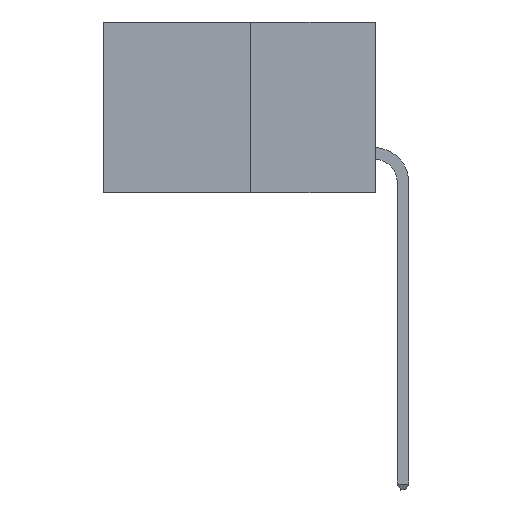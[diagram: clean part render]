
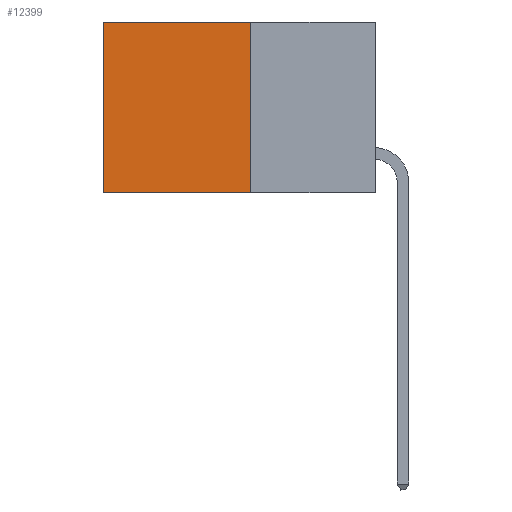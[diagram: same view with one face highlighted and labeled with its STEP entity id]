
A CAD part, left-side view. The second image highlights one B-rep face of the part: STEP entity #12399.
In plain terms, the highlighted planar face has unit normal (-1, 0, 0).
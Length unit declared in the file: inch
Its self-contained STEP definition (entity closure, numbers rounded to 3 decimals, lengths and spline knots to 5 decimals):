
#51 = LINE ( 'NONE', #8612, #17587 ) ;
#745 = FACE_OUTER_BOUND ( 'NONE', #1623, .T. ) ;
#1623 = EDGE_LOOP ( 'NONE', ( #15211, #9121, #4709, #14513 ) ) ;
#2615 = VERTEX_POINT ( 'NONE', #5876 ) ;
#2718 = VERTEX_POINT ( 'NONE', #7569 ) ;
#3143 = DIRECTION ( 'NONE',  ( 1., 0., 0. ) ) ;
#3274 = DIRECTION ( 'NONE',  ( 0., 1., 0. ) ) ;
#4709 = ORIENTED_EDGE ( 'NONE', *, *, #14621, .F. ) ;
#5876 = CARTESIAN_POINT ( 'NONE',  ( 0.277, 0.59, -0.37 ) ) ;
#6503 = CARTESIAN_POINT ( 'NONE',  ( 0.277, 0.59, -0.37 ) ) ;
#6609 = VECTOR ( 'NONE', #10995, 39.37008 ) ;
#7569 = CARTESIAN_POINT ( 'NONE',  ( 0.277, 0.27, -0.37 ) ) ;
#8198 = DIRECTION ( 'NONE',  ( 0., 0., -1. ) ) ;
#8321 = LINE ( 'NONE', #15035, #16805 ) ;
#8612 = CARTESIAN_POINT ( 'NONE',  ( 0.277, 0.27, 0. ) ) ;
#9121 = ORIENTED_EDGE ( 'NONE', *, *, #20484, .F. ) ;
#9159 = VERTEX_POINT ( 'NONE', #21028 ) ;
#10995 = DIRECTION ( 'NONE',  ( 0., 0., -1. ) ) ;
#11994 = DIRECTION ( 'NONE',  ( 0., 1., 0. ) ) ;
#12399 = ADVANCED_FACE ( 'NONE', ( #745 ), #20029, .F. ) ;
#13259 = CARTESIAN_POINT ( 'NONE',  ( 0.277, 0.27, -0.37 ) ) ;
#13660 = VECTOR ( 'NONE', #8198, 39.37008 ) ;
#14513 = ORIENTED_EDGE ( 'NONE', *, *, #18664, .T. ) ;
#14621 = EDGE_CURVE ( 'NONE', #21395, #2718, #20104, .T. ) ;
#14982 = DIRECTION ( 'NONE',  ( 0., 0., -1. ) ) ;
#15035 = CARTESIAN_POINT ( 'NONE',  ( 0.277, 0.27, -0.37 ) ) ;
#15211 = ORIENTED_EDGE ( 'NONE', *, *, #16924, .T. ) ;
#16805 = VECTOR ( 'NONE', #3274, 39.37008 ) ;
#16924 = EDGE_CURVE ( 'NONE', #9159, #2615, #18717, .T. ) ;
#17587 = VECTOR ( 'NONE', #11994, 39.37008 ) ;
#17857 = CARTESIAN_POINT ( 'NONE',  ( 0.277, 0.27, -0.37 ) ) ;
#18664 = EDGE_CURVE ( 'NONE', #21395, #9159, #51, .T. ) ;
#18717 = LINE ( 'NONE', #6503, #13660 ) ;
#20029 = PLANE ( 'NONE',  #20366 ) ;
#20104 = LINE ( 'NONE', #17857, #6609 ) ;
#20366 = AXIS2_PLACEMENT_3D ( 'NONE', #13259, #3143, #14982 ) ;
#20484 = EDGE_CURVE ( 'NONE', #2718, #2615, #8321, .T. ) ;
#20951 = CARTESIAN_POINT ( 'NONE',  ( 0.277, 0.27, 0. ) ) ;
#21028 = CARTESIAN_POINT ( 'NONE',  ( 0.277, 0.59, 0. ) ) ;
#21395 = VERTEX_POINT ( 'NONE', #20951 ) ;
